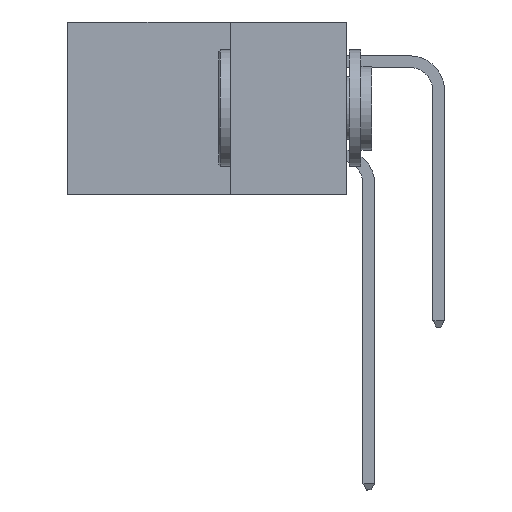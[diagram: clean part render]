
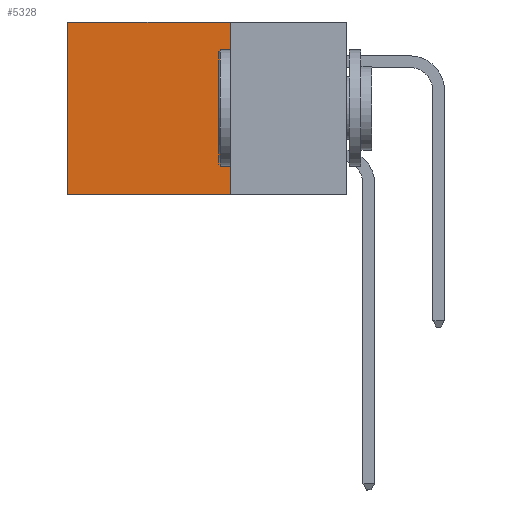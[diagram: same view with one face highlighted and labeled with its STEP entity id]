
A CAD part, left-side view. The second image highlights one B-rep face of the part: STEP entity #5328.
In plain terms, the highlighted planar face has unit normal (-1, 0, 0).
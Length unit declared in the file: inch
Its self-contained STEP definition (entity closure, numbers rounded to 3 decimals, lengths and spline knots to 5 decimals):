
#2494 = EDGE_CURVE ( 'NONE', #12494, #20829, #13165, .T. ) ;
#2874 = CARTESIAN_POINT ( 'NONE',  ( 0.2875, 0.25, 0. ) ) ;
#3708 = LINE ( 'NONE', #13670, #22432 ) ;
#3857 = CARTESIAN_POINT ( 'NONE',  ( 0.2875, 0.6, -0.37 ) ) ;
#5328 = ADVANCED_FACE ( 'NONE', ( #13743 ), #21607, .F. ) ;
#5924 = LINE ( 'NONE', #22923, #14405 ) ;
#6495 = CARTESIAN_POINT ( 'NONE',  ( 0.2875, 0.6, 0. ) ) ;
#6602 = VERTEX_POINT ( 'NONE', #6495 ) ;
#7623 = VECTOR ( 'NONE', #22154, 39.37008 ) ;
#8481 = DIRECTION ( 'NONE',  ( 0., 0., -1. ) ) ;
#9862 = EDGE_CURVE ( 'NONE', #12494, #6602, #3708, .T. ) ;
#10527 = ORIENTED_EDGE ( 'NONE', *, *, #9862, .T. ) ;
#11130 = EDGE_CURVE ( 'NONE', #6602, #15929, #5924, .T. ) ;
#12494 = VERTEX_POINT ( 'NONE', #17011 ) ;
#12571 = DIRECTION ( 'NONE',  ( 0., 0., -1. ) ) ;
#13165 = LINE ( 'NONE', #2874, #17987 ) ;
#13670 = CARTESIAN_POINT ( 'NONE',  ( 0.2875, 0.25, 0. ) ) ;
#13728 = DIRECTION ( 'NONE',  ( 0., 0., -1. ) ) ;
#13743 = FACE_OUTER_BOUND ( 'NONE', #21272, .T. ) ;
#14112 = EDGE_CURVE ( 'NONE', #20829, #15929, #18378, .T. ) ;
#14405 = VECTOR ( 'NONE', #8481, 39.37008 ) ;
#14929 = ORIENTED_EDGE ( 'NONE', *, *, #14112, .F. ) ;
#15509 = ORIENTED_EDGE ( 'NONE', *, *, #11130, .T. ) ;
#15732 = DIRECTION ( 'NONE',  ( 0., 1., 0. ) ) ;
#15929 = VERTEX_POINT ( 'NONE', #3857 ) ;
#16151 = CARTESIAN_POINT ( 'NONE',  ( 0.2875, 0.25, 0. ) ) ;
#17011 = CARTESIAN_POINT ( 'NONE',  ( 0.2875, 0.25, 0. ) ) ;
#17987 = VECTOR ( 'NONE', #13728, 39.37008 ) ;
#18378 = LINE ( 'NONE', #18402, #7623 ) ;
#18402 = CARTESIAN_POINT ( 'NONE',  ( 0.2875, 0.25, -0.37 ) ) ;
#18419 = AXIS2_PLACEMENT_3D ( 'NONE', #16151, #23459, #12571 ) ;
#20829 = VERTEX_POINT ( 'NONE', #23099 ) ;
#21272 = EDGE_LOOP ( 'NONE', ( #15509, #14929, #22582, #10527 ) ) ;
#21607 = PLANE ( 'NONE',  #18419 ) ;
#22154 = DIRECTION ( 'NONE',  ( 0., 1., 0. ) ) ;
#22432 = VECTOR ( 'NONE', #15732, 39.37008 ) ;
#22582 = ORIENTED_EDGE ( 'NONE', *, *, #2494, .F. ) ;
#22923 = CARTESIAN_POINT ( 'NONE',  ( 0.2875, 0.6, 0. ) ) ;
#23099 = CARTESIAN_POINT ( 'NONE',  ( 0.2875, 0.25, -0.37 ) ) ;
#23459 = DIRECTION ( 'NONE',  ( 1., 0., 0. ) ) ;
